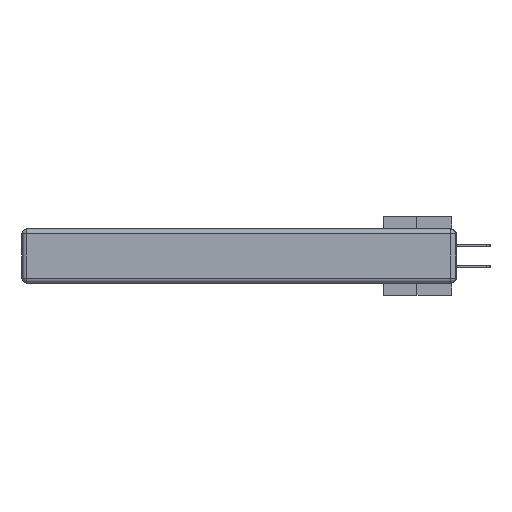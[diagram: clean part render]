
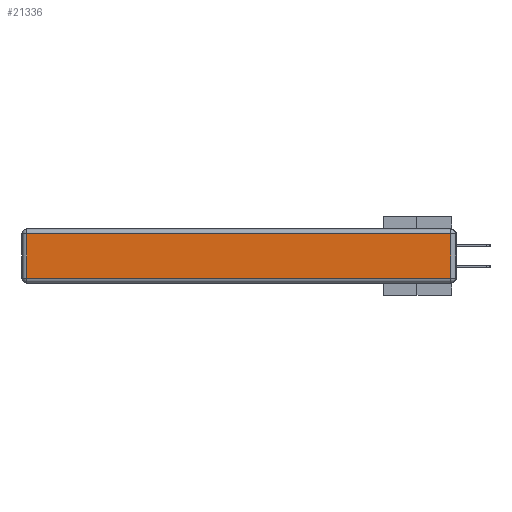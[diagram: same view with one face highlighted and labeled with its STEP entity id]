
A CAD part, left-side view. The second image highlights one B-rep face of the part: STEP entity #21336.
In plain terms, the highlighted planar face has unit normal (-1, 0, 0).
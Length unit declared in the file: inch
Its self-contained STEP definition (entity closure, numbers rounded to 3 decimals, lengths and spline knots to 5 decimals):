
#2988 = CARTESIAN_POINT ( 'NONE',  ( 0., 0., -0.343 ) ) ;
#4081 = CARTESIAN_POINT ( 'NONE',  ( 0., 2.72, -0.313 ) ) ;
#8350 = ORIENTED_EDGE ( 'NONE', *, *, #24153, .T. ) ;
#11283 = DIRECTION ( 'NONE',  ( 0., 1., 0. ) ) ;
#12049 = AXIS2_PLACEMENT_3D ( 'NONE', #2988, #19058, #41389 ) ;
#14634 = ORIENTED_EDGE ( 'NONE', *, *, #39867, .T. ) ;
#14702 = DIRECTION ( 'NONE',  ( 0., 0., -1. ) ) ;
#16431 = VECTOR ( 'NONE', #14702, 39.37008 ) ;
#17803 = LINE ( 'NONE', #31248, #32802 ) ;
#18379 = DIRECTION ( 'NONE',  ( 0., 0., 1. ) ) ;
#18515 = CARTESIAN_POINT ( 'NONE',  ( 0., 2.72, -0.03 ) ) ;
#18912 = EDGE_LOOP ( 'NONE', ( #39572, #14634, #8350, #38483 ) ) ;
#19058 = DIRECTION ( 'NONE',  ( -1., 0., 0. ) ) ;
#19350 = EDGE_CURVE ( 'NONE', #32056, #24418, #39046, .T. ) ;
#20182 = CARTESIAN_POINT ( 'NONE',  ( 0., 0., -0.313 ) ) ;
#21336 = ADVANCED_FACE ( 'NONE', ( #21357 ), #28432, .T. ) ;
#21357 = FACE_OUTER_BOUND ( 'NONE', #18912, .T. ) ;
#22551 = VECTOR ( 'NONE', #29980, 39.37008 ) ;
#24153 = EDGE_CURVE ( 'NONE', #35062, #31188, #38014, .T. ) ;
#24418 = VERTEX_POINT ( 'NONE', #30494 ) ;
#27433 = LINE ( 'NONE', #29818, #16431 ) ;
#28432 = PLANE ( 'NONE',  #12049 ) ;
#29306 = EDGE_CURVE ( 'NONE', #31188, #32056, #27433, .T. ) ;
#29818 = CARTESIAN_POINT ( 'NONE',  ( 0., 2.72, -0.343 ) ) ;
#29980 = DIRECTION ( 'NONE',  ( 0., -1., 0. ) ) ;
#30494 = CARTESIAN_POINT ( 'NONE',  ( 0., 0.03, -0.313 ) ) ;
#31188 = VERTEX_POINT ( 'NONE', #18515 ) ;
#31248 = CARTESIAN_POINT ( 'NONE',  ( 0., 0.03, -0.343 ) ) ;
#32056 = VERTEX_POINT ( 'NONE', #4081 ) ;
#32802 = VECTOR ( 'NONE', #18379, 39.37008 ) ;
#34525 = VECTOR ( 'NONE', #11283, 39.37008 ) ;
#35062 = VERTEX_POINT ( 'NONE', #38500 ) ;
#38014 = LINE ( 'NONE', #40075, #34525 ) ;
#38483 = ORIENTED_EDGE ( 'NONE', *, *, #29306, .T. ) ;
#38500 = CARTESIAN_POINT ( 'NONE',  ( 0., 0.03, -0.03 ) ) ;
#39046 = LINE ( 'NONE', #20182, #22551 ) ;
#39572 = ORIENTED_EDGE ( 'NONE', *, *, #19350, .T. ) ;
#39867 = EDGE_CURVE ( 'NONE', #24418, #35062, #17803, .T. ) ;
#40075 = CARTESIAN_POINT ( 'NONE',  ( 0., 2.75, -0.03 ) ) ;
#41389 = DIRECTION ( 'NONE',  ( 0., 0., 1. ) ) ;
